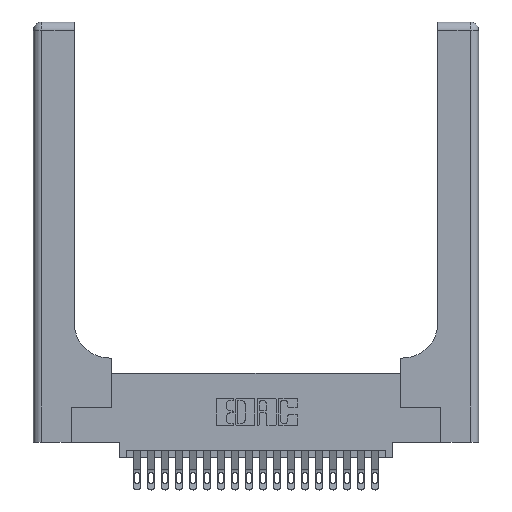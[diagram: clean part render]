
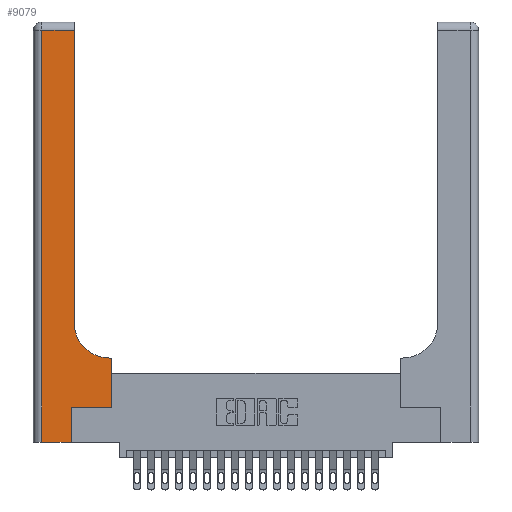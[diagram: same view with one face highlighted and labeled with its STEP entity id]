
A CAD part, top view. The second image highlights one B-rep face of the part: STEP entity #9079.
In plain terms, the highlighted planar face has unit normal (0, 0, 1).
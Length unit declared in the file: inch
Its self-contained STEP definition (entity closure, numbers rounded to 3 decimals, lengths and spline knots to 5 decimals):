
#128 = LINE ( 'NONE', #6657, #3497 ) ;
#1080 = CARTESIAN_POINT ( 'NONE',  ( 0.06, 0., 0.37 ) ) ;
#1154 = DIRECTION ( 'NONE',  ( 1., 0., 0. ) ) ;
#1207 = DIRECTION ( 'NONE',  ( 0., 1., 0. ) ) ;
#1294 = VECTOR ( 'NONE', #1154, 39.37008 ) ;
#1581 = CARTESIAN_POINT ( 'NONE',  ( 0., 2.94, 0.37 ) ) ;
#1852 = CARTESIAN_POINT ( 'NONE',  ( 0.06, 2.94, 0.37 ) ) ;
#1986 = CARTESIAN_POINT ( 'NONE',  ( 0.2915, 2.94, 0.37 ) ) ;
#2225 = VERTEX_POINT ( 'NONE', #1080 ) ;
#2445 = LINE ( 'NONE', #11754, #20770 ) ;
#2653 = CARTESIAN_POINT ( 'NONE',  ( 0., 3., 0.37 ) ) ;
#2816 = VECTOR ( 'NONE', #16820, 39.37008 ) ;
#2967 = DIRECTION ( 'NONE',  ( 0., 1., 0. ) ) ;
#2989 = LINE ( 'NONE', #1581, #22064 ) ;
#3011 = DIRECTION ( 'NONE',  ( 1., 0., 0. ) ) ;
#3497 = VECTOR ( 'NONE', #1207, 39.37008 ) ;
#3874 = VECTOR ( 'NONE', #2967, 39.37008 ) ;
#3971 = AXIS2_PLACEMENT_3D ( 'NONE', #2653, #13643, #16861 ) ;
#5063 = VERTEX_POINT ( 'NONE', #19431 ) ;
#5729 = CIRCLE ( 'NONE', #16709, 0.25 ) ;
#6101 = VERTEX_POINT ( 'NONE', #1852 ) ;
#6638 = CARTESIAN_POINT ( 'NONE',  ( 0.2915, 3., 0.37 ) ) ;
#6657 = CARTESIAN_POINT ( 'NONE',  ( 0.269, 0., 0.37 ) ) ;
#7655 = DIRECTION ( 'NONE',  ( 1., 0., 0. ) ) ;
#8125 = PLANE ( 'NONE',  #3971 ) ;
#8259 = VECTOR ( 'NONE', #17655, 39.37008 ) ;
#8326 = LINE ( 'NONE', #11553, #20522 ) ;
#8535 = EDGE_CURVE ( 'NONE', #18464, #9682, #128, .T. ) ;
#8671 = CARTESIAN_POINT ( 'NONE',  ( 0.2915, 0.6, 0.37 ) ) ;
#8744 = EDGE_CURVE ( 'NONE', #14252, #6101, #2989, .T. ) ;
#9079 = ADVANCED_FACE ( 'NONE', ( #22832 ), #8125, .F. ) ;
#9619 = ORIENTED_EDGE ( 'NONE', *, *, #17148, .T. ) ;
#9660 = CARTESIAN_POINT ( 'NONE',  ( 0.269, 0.25, 0.37 ) ) ;
#9682 = VERTEX_POINT ( 'NONE', #9660 ) ;
#9739 = LINE ( 'NONE', #6638, #3874 ) ;
#9898 = CARTESIAN_POINT ( 'NONE',  ( 0.269, 0.25, 0.37 ) ) ;
#11553 = CARTESIAN_POINT ( 'NONE',  ( 0.5585, 0.25, 0.37 ) ) ;
#11714 = DIRECTION ( 'NONE',  ( 0., 1., 0. ) ) ;
#11754 = CARTESIAN_POINT ( 'NONE',  ( 0., 0., 0.37 ) ) ;
#11959 = CARTESIAN_POINT ( 'NONE',  ( 0.5415, 0.6, 0.37 ) ) ;
#12041 = EDGE_CURVE ( 'NONE', #18087, #14252, #9739, .T. ) ;
#12127 = EDGE_LOOP ( 'NONE', ( #14119, #17962, #17261, #12662, #22153, #19984, #15092, #9619, #12515 ) ) ;
#12408 = DIRECTION ( 'NONE',  ( -1., 0., 0. ) ) ;
#12515 = ORIENTED_EDGE ( 'NONE', *, *, #17542, .T. ) ;
#12662 = ORIENTED_EDGE ( 'NONE', *, *, #16341, .T. ) ;
#12797 = VERTEX_POINT ( 'NONE', #11959 ) ;
#13643 = DIRECTION ( 'NONE',  ( 0., 0., -1. ) ) ;
#13880 = EDGE_CURVE ( 'NONE', #6101, #2225, #15081, .T. ) ;
#14119 = ORIENTED_EDGE ( 'NONE', *, *, #12041, .T. ) ;
#14252 = VERTEX_POINT ( 'NONE', #1986 ) ;
#14720 = VERTEX_POINT ( 'NONE', #22727 ) ;
#15081 = LINE ( 'NONE', #20328, #2816 ) ;
#15092 = ORIENTED_EDGE ( 'NONE', *, *, #22590, .T. ) ;
#16027 = LINE ( 'NONE', #8671, #8259 ) ;
#16341 = EDGE_CURVE ( 'NONE', #2225, #18464, #2445, .T. ) ;
#16709 = AXIS2_PLACEMENT_3D ( 'NONE', #20351, #18272, #7655 ) ;
#16820 = DIRECTION ( 'NONE',  ( 0., -1., 0. ) ) ;
#16861 = DIRECTION ( 'NONE',  ( -1., 0., 0. ) ) ;
#17148 = EDGE_CURVE ( 'NONE', #5063, #12797, #16027, .T. ) ;
#17261 = ORIENTED_EDGE ( 'NONE', *, *, #13880, .T. ) ;
#17542 = EDGE_CURVE ( 'NONE', #12797, #18087, #5729, .T. ) ;
#17646 = EDGE_CURVE ( 'NONE', #9682, #14720, #20200, .T. ) ;
#17655 = DIRECTION ( 'NONE',  ( -1., 0., 0. ) ) ;
#17962 = ORIENTED_EDGE ( 'NONE', *, *, #8744, .T. ) ;
#18087 = VERTEX_POINT ( 'NONE', #18622 ) ;
#18272 = DIRECTION ( 'NONE',  ( 0., 0., -1. ) ) ;
#18464 = VERTEX_POINT ( 'NONE', #21400 ) ;
#18622 = CARTESIAN_POINT ( 'NONE',  ( 0.2915, 0.85, 0.37 ) ) ;
#19431 = CARTESIAN_POINT ( 'NONE',  ( 0.5585, 0.6, 0.37 ) ) ;
#19984 = ORIENTED_EDGE ( 'NONE', *, *, #17646, .T. ) ;
#20200 = LINE ( 'NONE', #9898, #1294 ) ;
#20328 = CARTESIAN_POINT ( 'NONE',  ( 0.06, 3., 0.37 ) ) ;
#20351 = CARTESIAN_POINT ( 'NONE',  ( 0.5415, 0.85, 0.37 ) ) ;
#20522 = VECTOR ( 'NONE', #11714, 39.37008 ) ;
#20770 = VECTOR ( 'NONE', #3011, 39.37008 ) ;
#21400 = CARTESIAN_POINT ( 'NONE',  ( 0.269, 0., 0.37 ) ) ;
#22064 = VECTOR ( 'NONE', #12408, 39.37008 ) ;
#22153 = ORIENTED_EDGE ( 'NONE', *, *, #8535, .T. ) ;
#22590 = EDGE_CURVE ( 'NONE', #14720, #5063, #8326, .T. ) ;
#22727 = CARTESIAN_POINT ( 'NONE',  ( 0.5585, 0.25, 0.37 ) ) ;
#22832 = FACE_OUTER_BOUND ( 'NONE', #12127, .T. ) ;
